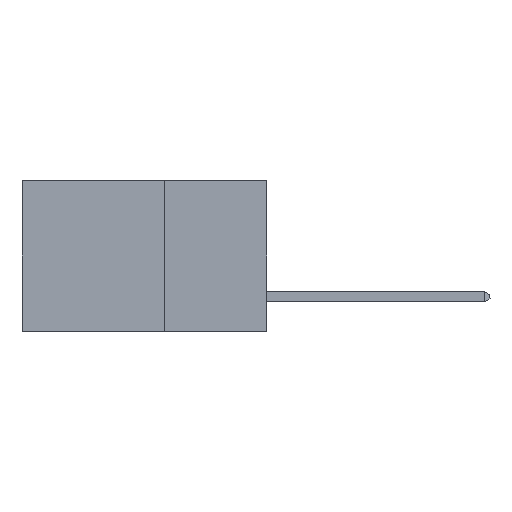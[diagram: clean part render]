
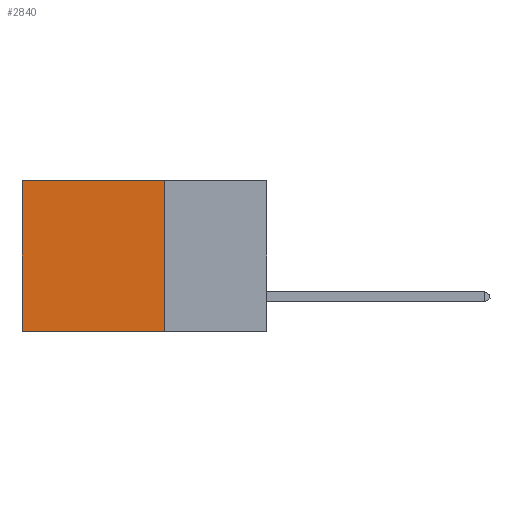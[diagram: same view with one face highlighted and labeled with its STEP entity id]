
A CAD part, left-side view. The second image highlights one B-rep face of the part: STEP entity #2840.
In plain terms, the highlighted planar face has unit normal (-1, 0, 0).
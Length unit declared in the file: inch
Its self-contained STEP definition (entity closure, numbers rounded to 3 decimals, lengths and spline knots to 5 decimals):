
#4 = CARTESIAN_POINT ( 'NONE',  ( 0.2875, 0.6, 0. ) ) ;
#796 = VECTOR ( 'NONE', #10975, 39.37008 ) ;
#1140 = LINE ( 'NONE', #12325, #796 ) ;
#1391 = VECTOR ( 'NONE', #12111, 39.37008 ) ;
#2403 = DIRECTION ( 'NONE',  ( 0., 1., 0. ) ) ;
#2594 = LINE ( 'NONE', #4, #11138 ) ;
#2657 = ORIENTED_EDGE ( 'NONE', *, *, #4898, .T. ) ;
#2777 = CARTESIAN_POINT ( 'NONE',  ( 0.2875, 0.6, -0.37 ) ) ;
#2840 = ADVANCED_FACE ( 'NONE', ( #12414 ), #5064, .F. ) ;
#3108 = CARTESIAN_POINT ( 'NONE',  ( 0.2875, 0.25, 0. ) ) ;
#3956 = EDGE_CURVE ( 'NONE', #5877, #7241, #9965, .T. ) ;
#3992 = EDGE_LOOP ( 'NONE', ( #2657, #4190, #5833, #8471 ) ) ;
#4190 = ORIENTED_EDGE ( 'NONE', *, *, #10683, .F. ) ;
#4898 = EDGE_CURVE ( 'NONE', #13809, #10139, #2594, .T. ) ;
#5053 = DIRECTION ( 'NONE',  ( 0., 0., -1. ) ) ;
#5062 = DIRECTION ( 'NONE',  ( 1., 0., 0. ) ) ;
#5064 = PLANE ( 'NONE',  #9324 ) ;
#5173 = CARTESIAN_POINT ( 'NONE',  ( 0.2875, 0.25, 0. ) ) ;
#5762 = CARTESIAN_POINT ( 'NONE',  ( 0.2875, 0.25, -0.37 ) ) ;
#5833 = ORIENTED_EDGE ( 'NONE', *, *, #3956, .F. ) ;
#5877 = VERTEX_POINT ( 'NONE', #3108 ) ;
#6323 = EDGE_CURVE ( 'NONE', #5877, #13809, #1140, .T. ) ;
#7241 = VERTEX_POINT ( 'NONE', #11727 ) ;
#8471 = ORIENTED_EDGE ( 'NONE', *, *, #6323, .T. ) ;
#9324 = AXIS2_PLACEMENT_3D ( 'NONE', #5173, #5062, #5053 ) ;
#9965 = LINE ( 'NONE', #11825, #1391 ) ;
#10139 = VERTEX_POINT ( 'NONE', #2777 ) ;
#10683 = EDGE_CURVE ( 'NONE', #7241, #10139, #11531, .T. ) ;
#10975 = DIRECTION ( 'NONE',  ( 0., 1., 0. ) ) ;
#11138 = VECTOR ( 'NONE', #13442, 39.37008 ) ;
#11531 = LINE ( 'NONE', #5762, #11882 ) ;
#11727 = CARTESIAN_POINT ( 'NONE',  ( 0.2875, 0.25, -0.37 ) ) ;
#11825 = CARTESIAN_POINT ( 'NONE',  ( 0.2875, 0.25, 0. ) ) ;
#11882 = VECTOR ( 'NONE', #2403, 39.37008 ) ;
#12111 = DIRECTION ( 'NONE',  ( 0., 0., -1. ) ) ;
#12325 = CARTESIAN_POINT ( 'NONE',  ( 0.2875, 0.25, 0. ) ) ;
#12414 = FACE_OUTER_BOUND ( 'NONE', #3992, .T. ) ;
#13099 = CARTESIAN_POINT ( 'NONE',  ( 0.2875, 0.6, 0. ) ) ;
#13442 = DIRECTION ( 'NONE',  ( 0., 0., -1. ) ) ;
#13809 = VERTEX_POINT ( 'NONE', #13099 ) ;
